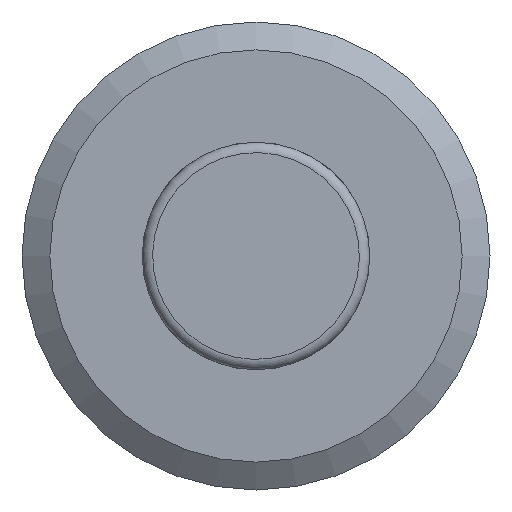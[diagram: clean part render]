
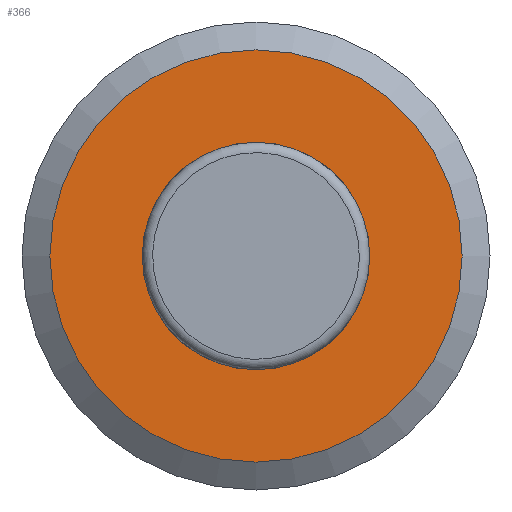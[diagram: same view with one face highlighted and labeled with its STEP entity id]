
A CAD part, front view. The second image highlights one B-rep face of the part: STEP entity #366.
In plain terms, the highlighted planar face has unit normal (0, -1, 0).
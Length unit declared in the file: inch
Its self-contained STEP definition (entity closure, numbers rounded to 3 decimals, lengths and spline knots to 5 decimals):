
#332=CARTESIAN_POINT('',(-0.0875,0.0,0.0));
#333=VERTEX_POINT('',#332);
#334=CARTESIAN_POINT('',(0.0,0.0,0.0));
#335=DIRECTION('',(0.0,1.0,0.0));
#336=DIRECTION('',(-1.0,0.0,0.0));
#337=AXIS2_PLACEMENT_3D('',#334,#335,#336);
#338=CIRCLE('',#337,0.0875);
#339=EDGE_CURVE('',#333,#333,#338,.T.);
#347=CARTESIAN_POINT('',(-0.12299,0.,0.0));
#348=DIRECTION('',(0.0,-1.0,0.0));
#349=DIRECTION('',(0.0,0.0,-1.0));
#350=AXIS2_PLACEMENT_3D('',#347,#348,#349);
#351=PLANE('',#350);
#352=CARTESIAN_POINT('',(-0.15848,0.,0.0));
#353=VERTEX_POINT('',#352);
#354=CARTESIAN_POINT('',(0.0,0.0,0.0));
#355=DIRECTION('',(0.0,1.0,0.0));
#356=DIRECTION('',(-1.0,0.0,0.0));
#357=AXIS2_PLACEMENT_3D('',#354,#355,#356);
#358=CIRCLE('',#357,0.15848);
#359=EDGE_CURVE('',#353,#353,#358,.T.);
#360=ORIENTED_EDGE('',*,*,#359,.F.);
#361=EDGE_LOOP('',(#360));
#362=FACE_OUTER_BOUND('',#361,.T.);
#363=ORIENTED_EDGE('',*,*,#339,.T.);
#364=EDGE_LOOP('',(#363));
#365=FACE_BOUND('',#364,.T.);
#366=ADVANCED_FACE('',(#362,#365),#351,.T.);
